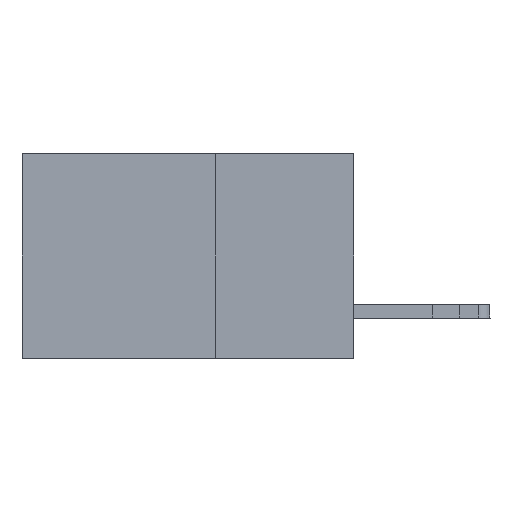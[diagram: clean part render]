
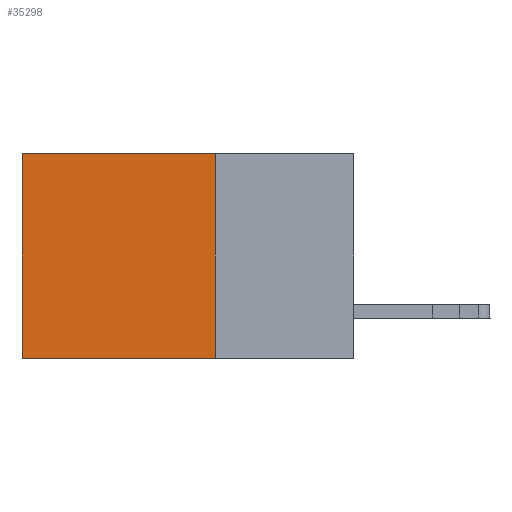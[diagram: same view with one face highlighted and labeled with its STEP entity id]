
A CAD part, left-side view. The second image highlights one B-rep face of the part: STEP entity #35298.
In plain terms, the highlighted planar face has unit normal (-1, 0, 0).
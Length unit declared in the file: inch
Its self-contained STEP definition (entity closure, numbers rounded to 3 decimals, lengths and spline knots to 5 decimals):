
#3046 = ORIENTED_EDGE ( 'NONE', *, *, #29135, .T. ) ;
#3099 = LINE ( 'NONE', #11243, #31571 ) ;
#3916 = LINE ( 'NONE', #12764, #10537 ) ;
#4126 = VERTEX_POINT ( 'NONE', #28313 ) ;
#4478 = CARTESIAN_POINT ( 'NONE',  ( 0.2875, 0.25, 0. ) ) ;
#5596 = VECTOR ( 'NONE', #23343, 39.37008 ) ;
#8090 = EDGE_CURVE ( 'NONE', #21677, #31941, #21147, .T. ) ;
#8727 = LINE ( 'NONE', #24803, #23338 ) ;
#8818 = FACE_OUTER_BOUND ( 'NONE', #13284, .T. ) ;
#9637 = ORIENTED_EDGE ( 'NONE', *, *, #29992, .F. ) ;
#10537 = VECTOR ( 'NONE', #34594, 39.37008 ) ;
#11243 = CARTESIAN_POINT ( 'NONE',  ( 0.2875, 0.6, 0. ) ) ;
#12764 = CARTESIAN_POINT ( 'NONE',  ( 0.2875, 0.25, -0.37 ) ) ;
#13284 = EDGE_LOOP ( 'NONE', ( #3046, #9637, #22853, #15588 ) ) ;
#14028 = DIRECTION ( 'NONE',  ( 0., 0., -1. ) ) ;
#15588 = ORIENTED_EDGE ( 'NONE', *, *, #8090, .T. ) ;
#16837 = AXIS2_PLACEMENT_3D ( 'NONE', #35678, #30328, #14028 ) ;
#17871 = CARTESIAN_POINT ( 'NONE',  ( 0.2875, 0.25, 0. ) ) ;
#18579 = EDGE_CURVE ( 'NONE', #21677, #4126, #8727, .T. ) ;
#21147 = LINE ( 'NONE', #17871, #5596 ) ;
#21677 = VERTEX_POINT ( 'NONE', #4478 ) ;
#22853 = ORIENTED_EDGE ( 'NONE', *, *, #18579, .F. ) ;
#23338 = VECTOR ( 'NONE', #35629, 39.37008 ) ;
#23343 = DIRECTION ( 'NONE',  ( 0., 1., 0. ) ) ;
#24803 = CARTESIAN_POINT ( 'NONE',  ( 0.2875, 0.25, 0. ) ) ;
#24956 = DIRECTION ( 'NONE',  ( 0., 0., -1. ) ) ;
#27530 = PLANE ( 'NONE',  #16837 ) ;
#28313 = CARTESIAN_POINT ( 'NONE',  ( 0.2875, 0.25, -0.37 ) ) ;
#29135 = EDGE_CURVE ( 'NONE', #31941, #30168, #3099, .T. ) ;
#29992 = EDGE_CURVE ( 'NONE', #4126, #30168, #3916, .T. ) ;
#30168 = VERTEX_POINT ( 'NONE', #33052 ) ;
#30328 = DIRECTION ( 'NONE',  ( 1., 0., 0. ) ) ;
#31571 = VECTOR ( 'NONE', #24956, 39.37008 ) ;
#31941 = VERTEX_POINT ( 'NONE', #35166 ) ;
#33052 = CARTESIAN_POINT ( 'NONE',  ( 0.2875, 0.6, -0.37 ) ) ;
#34594 = DIRECTION ( 'NONE',  ( 0., 1., 0. ) ) ;
#35166 = CARTESIAN_POINT ( 'NONE',  ( 0.2875, 0.6, 0. ) ) ;
#35298 = ADVANCED_FACE ( 'NONE', ( #8818 ), #27530, .F. ) ;
#35629 = DIRECTION ( 'NONE',  ( 0., 0., -1. ) ) ;
#35678 = CARTESIAN_POINT ( 'NONE',  ( 0.2875, 0.25, 0. ) ) ;
